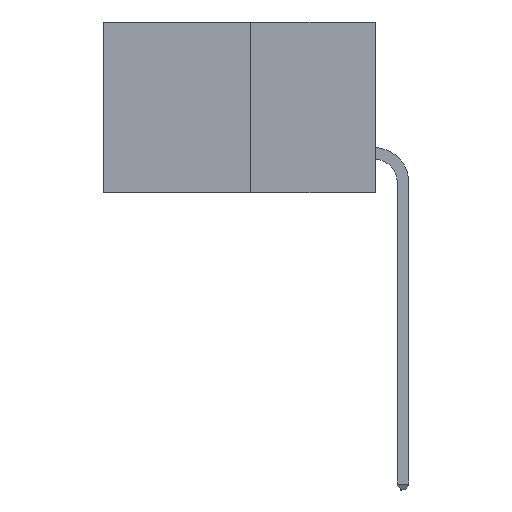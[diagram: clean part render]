
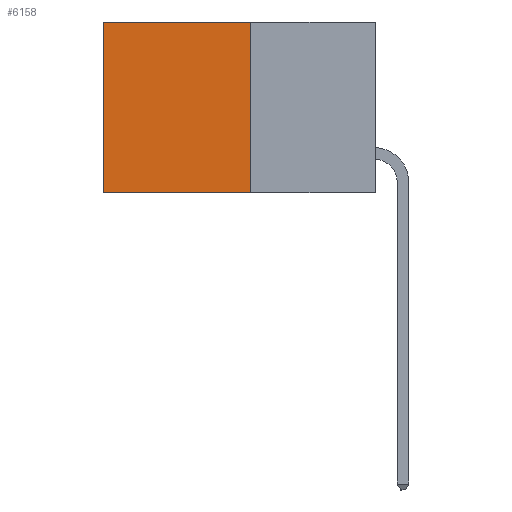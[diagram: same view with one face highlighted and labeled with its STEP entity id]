
A CAD part, left-side view. The second image highlights one B-rep face of the part: STEP entity #6158.
In plain terms, the highlighted planar face has unit normal (-1, 0, 0).
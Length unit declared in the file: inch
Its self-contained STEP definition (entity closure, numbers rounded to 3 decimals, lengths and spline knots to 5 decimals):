
#29 = CARTESIAN_POINT ( 'NONE',  ( 0.277, 0.27, -0.37 ) ) ;
#1180 = LINE ( 'NONE', #5152, #10836 ) ;
#1653 = VERTEX_POINT ( 'NONE', #5143 ) ;
#1713 = DIRECTION ( 'NONE',  ( 0., 0., -1. ) ) ;
#1945 = VERTEX_POINT ( 'NONE', #3567 ) ;
#2414 = VECTOR ( 'NONE', #8199, 39.37008 ) ;
#2448 = LINE ( 'NONE', #6300, #7043 ) ;
#2731 = CARTESIAN_POINT ( 'NONE',  ( 0.277, 0.27, 0. ) ) ;
#2920 = DIRECTION ( 'NONE',  ( 0., 1., 0. ) ) ;
#3567 = CARTESIAN_POINT ( 'NONE',  ( 0.277, 0.59, 0. ) ) ;
#4215 = DIRECTION ( 'NONE',  ( 0., 0., -1. ) ) ;
#4624 = DIRECTION ( 'NONE',  ( 1., 0., 0. ) ) ;
#4967 = VERTEX_POINT ( 'NONE', #6509 ) ;
#5143 = CARTESIAN_POINT ( 'NONE',  ( 0.277, 0.27, -0.37 ) ) ;
#5152 = CARTESIAN_POINT ( 'NONE',  ( 0.277, 0.27, -0.37 ) ) ;
#5365 = ORIENTED_EDGE ( 'NONE', *, *, #6135, .T. ) ;
#5492 = ORIENTED_EDGE ( 'NONE', *, *, #11533, .F. ) ;
#5576 = ORIENTED_EDGE ( 'NONE', *, *, #6908, .F. ) ;
#5589 = AXIS2_PLACEMENT_3D ( 'NONE', #9113, #4624, #10878 ) ;
#5886 = ORIENTED_EDGE ( 'NONE', *, *, #8577, .T. ) ;
#6135 = EDGE_CURVE ( 'NONE', #4967, #1945, #7580, .T. ) ;
#6158 = ADVANCED_FACE ( 'NONE', ( #9352 ), #8236, .F. ) ;
#6300 = CARTESIAN_POINT ( 'NONE',  ( 0.277, 0.59, -0.37 ) ) ;
#6509 = CARTESIAN_POINT ( 'NONE',  ( 0.277, 0.27, 0. ) ) ;
#6908 = EDGE_CURVE ( 'NONE', #1653, #7300, #9209, .T. ) ;
#7043 = VECTOR ( 'NONE', #1713, 39.37008 ) ;
#7300 = VERTEX_POINT ( 'NONE', #8885 ) ;
#7580 = LINE ( 'NONE', #2731, #2414 ) ;
#8137 = EDGE_LOOP ( 'NONE', ( #5886, #5576, #5492, #5365 ) ) ;
#8199 = DIRECTION ( 'NONE',  ( 0., 1., 0. ) ) ;
#8236 = PLANE ( 'NONE',  #5589 ) ;
#8577 = EDGE_CURVE ( 'NONE', #1945, #7300, #2448, .T. ) ;
#8885 = CARTESIAN_POINT ( 'NONE',  ( 0.277, 0.59, -0.37 ) ) ;
#9113 = CARTESIAN_POINT ( 'NONE',  ( 0.277, 0.27, -0.37 ) ) ;
#9209 = LINE ( 'NONE', #29, #10995 ) ;
#9352 = FACE_OUTER_BOUND ( 'NONE', #8137, .T. ) ;
#10836 = VECTOR ( 'NONE', #4215, 39.37008 ) ;
#10878 = DIRECTION ( 'NONE',  ( 0., 0., -1. ) ) ;
#10995 = VECTOR ( 'NONE', #2920, 39.37008 ) ;
#11533 = EDGE_CURVE ( 'NONE', #4967, #1653, #1180, .T. ) ;
